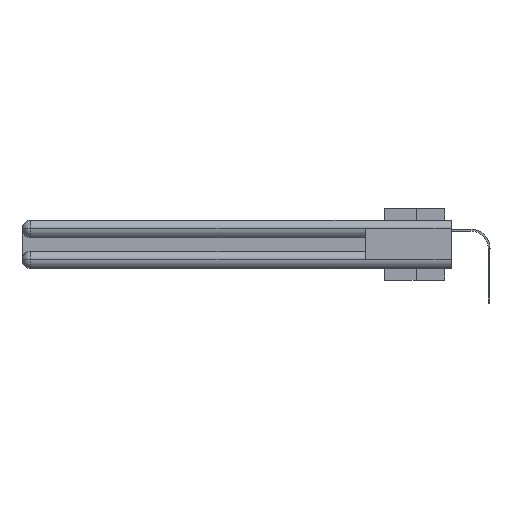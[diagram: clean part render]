
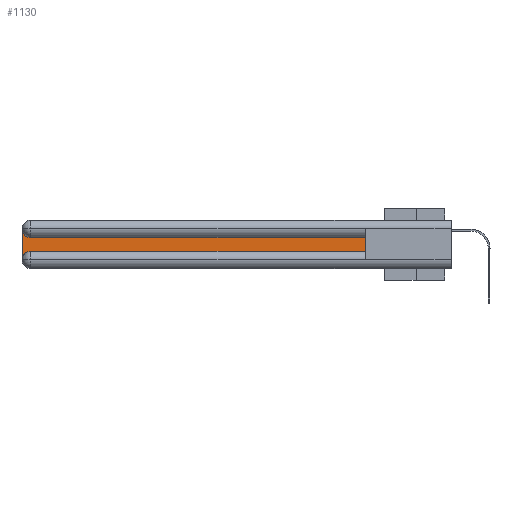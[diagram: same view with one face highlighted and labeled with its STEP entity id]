
A CAD part, left-side view. The second image highlights one B-rep face of the part: STEP entity #1130.
In plain terms, the highlighted planar face has unit normal (-1, 0, 0).
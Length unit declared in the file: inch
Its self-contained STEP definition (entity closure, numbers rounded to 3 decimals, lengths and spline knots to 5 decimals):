
#1062 = DIRECTION ( 'NONE',  ( 1., 0., 0. ) ) ;
#1130 = ADVANCED_FACE ( 'NONE', ( #1381 ), #21238, .F. ) ;
#1330 = CARTESIAN_POINT ( 'NONE',  ( 0.075, 3., -0.2175 ) ) ;
#1381 = FACE_OUTER_BOUND ( 'NONE', #29217, .T. ) ;
#1815 = CARTESIAN_POINT ( 'NONE',  ( 0.075, 2.94, -0.1225 ) ) ;
#2240 = AXIS2_PLACEMENT_3D ( 'NONE', #18803, #1062, #11454 ) ;
#3055 = DIRECTION ( 'NONE',  ( 0., 0., -1. ) ) ;
#3553 = ORIENTED_EDGE ( 'NONE', *, *, #12552, .T. ) ;
#3949 = CARTESIAN_POINT ( 'NONE',  ( 0.075, 3., -0.0625 ) ) ;
#5897 = VERTEX_POINT ( 'NONE', #23105 ) ;
#6312 = CIRCLE ( 'NONE', #26085, 0.06 ) ;
#6383 = CARTESIAN_POINT ( 'NONE',  ( 0.075, 0.6, -0.1225 ) ) ;
#6968 = LINE ( 'NONE', #31559, #24397 ) ;
#8236 = VERTEX_POINT ( 'NONE', #13567 ) ;
#8643 = EDGE_CURVE ( 'NONE', #15599, #17380, #6968, .T. ) ;
#10271 = CARTESIAN_POINT ( 'NONE',  ( 0.075, 0.6, -0.2175 ) ) ;
#10435 = AXIS2_PLACEMENT_3D ( 'NONE', #29810, #26891, #19725 ) ;
#10673 = ORIENTED_EDGE ( 'NONE', *, *, #22741, .T. ) ;
#11245 = DIRECTION ( 'NONE',  ( 0., 0., -1. ) ) ;
#11454 = DIRECTION ( 'NONE',  ( 0., 0., -1. ) ) ;
#12161 = VERTEX_POINT ( 'NONE', #3949 ) ;
#12552 = EDGE_CURVE ( 'NONE', #12161, #5897, #21184, .T. ) ;
#13567 = CARTESIAN_POINT ( 'NONE',  ( 0.075, 2.94, -0.2175 ) ) ;
#14102 = VERTEX_POINT ( 'NONE', #19266 ) ;
#15599 = VERTEX_POINT ( 'NONE', #6383 ) ;
#16980 = EDGE_CURVE ( 'NONE', #14102, #15599, #17132, .T. ) ;
#17132 = LINE ( 'NONE', #10271, #27355 ) ;
#17380 = VERTEX_POINT ( 'NONE', #1815 ) ;
#17881 = CARTESIAN_POINT ( 'NONE',  ( 0.075, 2.94, -0.0625 ) ) ;
#18703 = CARTESIAN_POINT ( 'NONE',  ( 0.075, 0.6, -0.2175 ) ) ;
#18803 = CARTESIAN_POINT ( 'NONE',  ( 0.075, 3., -0.1225 ) ) ;
#19266 = CARTESIAN_POINT ( 'NONE',  ( 0.075, 0.6, -0.2175 ) ) ;
#19406 = ORIENTED_EDGE ( 'NONE', *, *, #29680, .T. ) ;
#19725 = DIRECTION ( 'NONE',  ( 0., 0., -1. ) ) ;
#20141 = DIRECTION ( 'NONE',  ( 1., 0., 0. ) ) ;
#20737 = ORIENTED_EDGE ( 'NONE', *, *, #16980, .T. ) ;
#21184 = LINE ( 'NONE', #1330, #31527 ) ;
#21238 = PLANE ( 'NONE',  #2240 ) ;
#21616 = DIRECTION ( 'NONE',  ( 0., -1., 0. ) ) ;
#22741 = EDGE_CURVE ( 'NONE', #8236, #14102, #26489, .T. ) ;
#23040 = CIRCLE ( 'NONE', #10435, 0.06 ) ;
#23105 = CARTESIAN_POINT ( 'NONE',  ( 0.075, 3., -0.2775 ) ) ;
#23281 = ORIENTED_EDGE ( 'NONE', *, *, #8643, .T. ) ;
#24397 = VECTOR ( 'NONE', #29122, 39.37008 ) ;
#26085 = AXIS2_PLACEMENT_3D ( 'NONE', #17881, #20141, #3055 ) ;
#26489 = LINE ( 'NONE', #18703, #31865 ) ;
#26891 = DIRECTION ( 'NONE',  ( 1., 0., 0. ) ) ;
#27355 = VECTOR ( 'NONE', #27547, 39.37008 ) ;
#27547 = DIRECTION ( 'NONE',  ( 0., 0., 1. ) ) ;
#29122 = DIRECTION ( 'NONE',  ( 0., 1., 0. ) ) ;
#29217 = EDGE_LOOP ( 'NONE', ( #23281, #32034, #3553, #19406, #10673, #20737 ) ) ;
#29680 = EDGE_CURVE ( 'NONE', #5897, #8236, #23040, .T. ) ;
#29810 = CARTESIAN_POINT ( 'NONE',  ( 0.075, 2.94, -0.2775 ) ) ;
#31527 = VECTOR ( 'NONE', #11245, 39.37008 ) ;
#31559 = CARTESIAN_POINT ( 'NONE',  ( 0.075, 0.6, -0.1225 ) ) ;
#31865 = VECTOR ( 'NONE', #21616, 39.37008 ) ;
#32034 = ORIENTED_EDGE ( 'NONE', *, *, #32075, .T. ) ;
#32075 = EDGE_CURVE ( 'NONE', #17380, #12161, #6312, .T. ) ;
